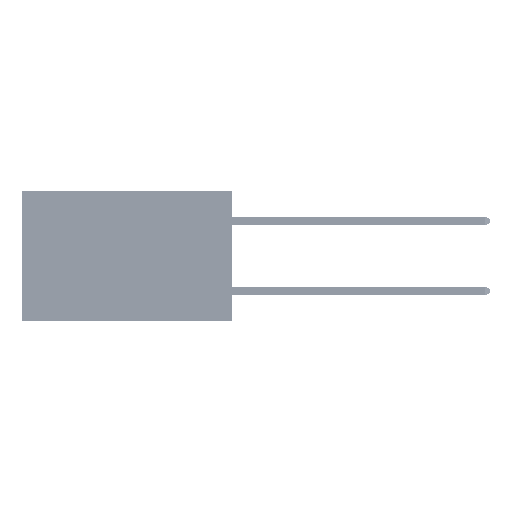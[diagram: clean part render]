
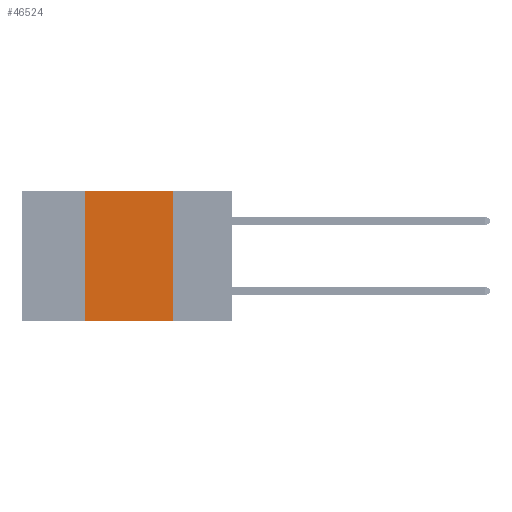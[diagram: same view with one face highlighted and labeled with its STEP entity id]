
A CAD part, left-side view. The second image highlights one B-rep face of the part: STEP entity #46524.
In plain terms, the highlighted planar face has unit normal (-1, 0, 0).
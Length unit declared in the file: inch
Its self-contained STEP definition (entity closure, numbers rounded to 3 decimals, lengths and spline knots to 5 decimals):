
#2449 = ORIENTED_EDGE ( 'NONE', *, *, #31204, .F. ) ;
#3127 = LINE ( 'NONE', #39192, #45502 ) ;
#5394 = VERTEX_POINT ( 'NONE', #16505 ) ;
#5750 = EDGE_CURVE ( 'NONE', #31580, #5394, #30854, .T. ) ;
#6701 = EDGE_LOOP ( 'NONE', ( #30792, #2449, #6714, #24802 ) ) ;
#6714 = ORIENTED_EDGE ( 'NONE', *, *, #5750, .F. ) ;
#8640 = CARTESIAN_POINT ( 'NONE',  ( 0., 0.6, 0. ) ) ;
#10760 = VECTOR ( 'NONE', #39308, 39.37008 ) ;
#11750 = EDGE_CURVE ( 'NONE', #19399, #27797, #30501, .T. ) ;
#12686 = CARTESIAN_POINT ( 'NONE',  ( 0., 0.17, 0. ) ) ;
#16365 = PLANE ( 'NONE',  #32602 ) ;
#16505 = CARTESIAN_POINT ( 'NONE',  ( 0., 0.42, 0. ) ) ;
#17454 = VECTOR ( 'NONE', #34437, 39.37008 ) ;
#17706 = FACE_OUTER_BOUND ( 'NONE', #6701, .T. ) ;
#19399 = VERTEX_POINT ( 'NONE', #12686 ) ;
#20068 = DIRECTION ( 'NONE',  ( 0., 0., -1. ) ) ;
#23197 = CARTESIAN_POINT ( 'NONE',  ( 0., 0.6, 0. ) ) ;
#24802 = ORIENTED_EDGE ( 'NONE', *, *, #42127, .T. ) ;
#26264 = CARTESIAN_POINT ( 'NONE',  ( 0., 0.42, 0. ) ) ;
#27797 = VERTEX_POINT ( 'NONE', #37062 ) ;
#30501 = LINE ( 'NONE', #42476, #31792 ) ;
#30792 = ORIENTED_EDGE ( 'NONE', *, *, #11750, .F. ) ;
#30854 = LINE ( 'NONE', #26264, #17454 ) ;
#31204 = EDGE_CURVE ( 'NONE', #5394, #19399, #32347, .T. ) ;
#31580 = VERTEX_POINT ( 'NONE', #38565 ) ;
#31792 = VECTOR ( 'NONE', #34564, 39.37008 ) ;
#32347 = LINE ( 'NONE', #23197, #10760 ) ;
#32602 = AXIS2_PLACEMENT_3D ( 'NONE', #8640, #36916, #20068 ) ;
#34437 = DIRECTION ( 'NONE',  ( 0., 0., 1. ) ) ;
#34564 = DIRECTION ( 'NONE',  ( 0., 0., -1. ) ) ;
#36916 = DIRECTION ( 'NONE',  ( 1., 0., 0. ) ) ;
#37062 = CARTESIAN_POINT ( 'NONE',  ( 0., 0.17, -0.37 ) ) ;
#38565 = CARTESIAN_POINT ( 'NONE',  ( 0., 0.42, -0.37 ) ) ;
#39192 = CARTESIAN_POINT ( 'NONE',  ( 0., 0.6, -0.37 ) ) ;
#39308 = DIRECTION ( 'NONE',  ( 0., -1., 0. ) ) ;
#42127 = EDGE_CURVE ( 'NONE', #31580, #27797, #3127, .T. ) ;
#42476 = CARTESIAN_POINT ( 'NONE',  ( 0., 0.17, 0. ) ) ;
#45502 = VECTOR ( 'NONE', #51186, 39.37008 ) ;
#46524 = ADVANCED_FACE ( 'NONE', ( #17706 ), #16365, .F. ) ;
#51186 = DIRECTION ( 'NONE',  ( 0., -1., 0. ) ) ;
